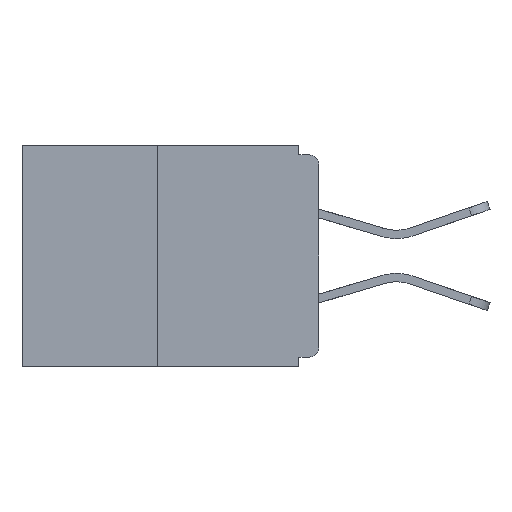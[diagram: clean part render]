
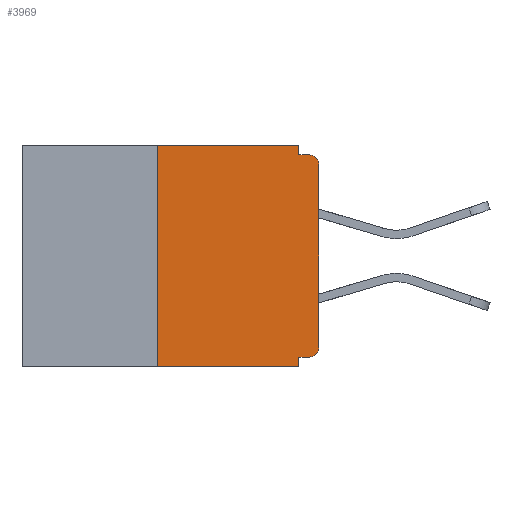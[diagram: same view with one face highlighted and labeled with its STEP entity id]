
A CAD part, left-side view. The second image highlights one B-rep face of the part: STEP entity #3969.
In plain terms, the highlighted planar face has unit normal (-1, 0, 0).
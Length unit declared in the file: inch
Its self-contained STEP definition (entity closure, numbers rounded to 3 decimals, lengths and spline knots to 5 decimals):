
#8 = VERTEX_POINT ( 'NONE', #7921 ) ;
#46 = ORIENTED_EDGE ( 'NONE', *, *, #6906, .F. ) ;
#98 = EDGE_CURVE ( 'NONE', #11477, #3747, #10595, .T. ) ;
#125 = VECTOR ( 'NONE', #12243, 39.37008 ) ;
#426 = DIRECTION ( 'NONE',  ( 0., 0., -1. ) ) ;
#535 = VERTEX_POINT ( 'NONE', #3699 ) ;
#546 = CARTESIAN_POINT ( 'NONE',  ( 0., 0.25, -0.343 ) ) ;
#581 = LINE ( 'NONE', #2381, #2431 ) ;
#599 = ORIENTED_EDGE ( 'NONE', *, *, #8883, .T. ) ;
#720 = EDGE_LOOP ( 'NONE', ( #8506, #5091, #4333, #13013, #10752, #8217, #8683, #599, #46, #11203 ) ) ;
#773 = CARTESIAN_POINT ( 'NONE',  ( 0., 0.25, 0. ) ) ;
#1029 = VECTOR ( 'NONE', #7356, 39.37008 ) ;
#1056 = CARTESIAN_POINT ( 'NONE',  ( 0., 0.46, 0. ) ) ;
#1075 = VECTOR ( 'NONE', #1654, 39.37008 ) ;
#1450 = LINE ( 'NONE', #6762, #2303 ) ;
#1654 = DIRECTION ( 'NONE',  ( 0., 0., -1. ) ) ;
#1797 = AXIS2_PLACEMENT_3D ( 'NONE', #3157, #8465, #10649 ) ;
#2116 = DIRECTION ( 'NONE',  ( -1., 0., 0. ) ) ;
#2211 = CARTESIAN_POINT ( 'NONE',  ( 0., 0.015, -0.03 ) ) ;
#2303 = VECTOR ( 'NONE', #5671, 39.37008 ) ;
#2381 = CARTESIAN_POINT ( 'NONE',  ( 0., 0.46, 0. ) ) ;
#2431 = VECTOR ( 'NONE', #8765, 39.37008 ) ;
#2503 = AXIS2_PLACEMENT_3D ( 'NONE', #1056, #4284, #10712 ) ;
#2799 = EDGE_CURVE ( 'NONE', #5408, #12318, #581, .T. ) ;
#3157 = CARTESIAN_POINT ( 'NONE',  ( 0., 0.015, -0.313 ) ) ;
#3571 = VECTOR ( 'NONE', #8159, 39.37008 ) ;
#3699 = CARTESIAN_POINT ( 'NONE',  ( 0., 0.031, -0.343 ) ) ;
#3747 = VERTEX_POINT ( 'NONE', #12670 ) ;
#3969 = ADVANCED_FACE ( 'NONE', ( #12938 ), #10816, .F. ) ;
#4093 = CARTESIAN_POINT ( 'NONE',  ( 0., 0.031, -0.328 ) ) ;
#4284 = DIRECTION ( 'NONE',  ( 1., 0., 0. ) ) ;
#4333 = ORIENTED_EDGE ( 'NONE', *, *, #10765, .T. ) ;
#4395 = DIRECTION ( 'NONE',  ( 0., 0., -1. ) ) ;
#4459 = AXIS2_PLACEMENT_3D ( 'NONE', #2211, #2116, #4395 ) ;
#4701 = CARTESIAN_POINT ( 'NONE',  ( 0., 0.015, -0.015 ) ) ;
#4711 = EDGE_CURVE ( 'NONE', #6482, #535, #12909, .T. ) ;
#4891 = CARTESIAN_POINT ( 'NONE',  ( 0., 0., 0. ) ) ;
#5045 = CIRCLE ( 'NONE', #4459, 0.015 ) ;
#5091 = ORIENTED_EDGE ( 'NONE', *, *, #6519, .F. ) ;
#5249 = DIRECTION ( 'NONE',  ( 0., 0., 1. ) ) ;
#5408 = VERTEX_POINT ( 'NONE', #773 ) ;
#5530 = LINE ( 'NONE', #6196, #8367 ) ;
#5671 = DIRECTION ( 'NONE',  ( 0., -1., 0. ) ) ;
#6196 = CARTESIAN_POINT ( 'NONE',  ( 0., 0.25, 0. ) ) ;
#6482 = VERTEX_POINT ( 'NONE', #4093 ) ;
#6519 = EDGE_CURVE ( 'NONE', #11495, #5408, #5530, .T. ) ;
#6762 = CARTESIAN_POINT ( 'NONE',  ( 0., 0.46, -0.343 ) ) ;
#6906 = EDGE_CURVE ( 'NONE', #8, #9247, #12513, .T. ) ;
#7252 = VECTOR ( 'NONE', #426, 39.37008 ) ;
#7356 = DIRECTION ( 'NONE',  ( 0., 1., 0. ) ) ;
#7921 = CARTESIAN_POINT ( 'NONE',  ( 0., 0.031, -0.015 ) ) ;
#8069 = CARTESIAN_POINT ( 'NONE',  ( 0., 0.031, 0. ) ) ;
#8094 = LINE ( 'NONE', #11783, #1029 ) ;
#8159 = DIRECTION ( 'NONE',  ( 0., 0., 1. ) ) ;
#8217 = ORIENTED_EDGE ( 'NONE', *, *, #13290, .T. ) ;
#8367 = VECTOR ( 'NONE', #5249, 39.37008 ) ;
#8465 = DIRECTION ( 'NONE',  ( -1., 0., 0. ) ) ;
#8506 = ORIENTED_EDGE ( 'NONE', *, *, #2799, .F. ) ;
#8683 = ORIENTED_EDGE ( 'NONE', *, *, #98, .T. ) ;
#8765 = DIRECTION ( 'NONE',  ( 0., -1., 0. ) ) ;
#8883 = EDGE_CURVE ( 'NONE', #3747, #9247, #5045, .T. ) ;
#8965 = CARTESIAN_POINT ( 'NONE',  ( 0., 0.031, -0.343 ) ) ;
#8981 = VERTEX_POINT ( 'NONE', #11478 ) ;
#9143 = LINE ( 'NONE', #8069, #1075 ) ;
#9247 = VERTEX_POINT ( 'NONE', #4701 ) ;
#10492 = CIRCLE ( 'NONE', #1797, 0.015 ) ;
#10595 = LINE ( 'NONE', #4891, #3571 ) ;
#10649 = DIRECTION ( 'NONE',  ( 0., 0., -1. ) ) ;
#10712 = DIRECTION ( 'NONE',  ( 0., 0., -1. ) ) ;
#10752 = ORIENTED_EDGE ( 'NONE', *, *, #12828, .F. ) ;
#10765 = EDGE_CURVE ( 'NONE', #11495, #535, #1450, .T. ) ;
#10816 = PLANE ( 'NONE',  #2503 ) ;
#11172 = CARTESIAN_POINT ( 'NONE',  ( 0., 0., -0.015 ) ) ;
#11203 = ORIENTED_EDGE ( 'NONE', *, *, #11877, .F. ) ;
#11477 = VERTEX_POINT ( 'NONE', #13274 ) ;
#11478 = CARTESIAN_POINT ( 'NONE',  ( 0., 0.015, -0.328 ) ) ;
#11495 = VERTEX_POINT ( 'NONE', #546 ) ;
#11783 = CARTESIAN_POINT ( 'NONE',  ( 0., 0., -0.328 ) ) ;
#11877 = EDGE_CURVE ( 'NONE', #12318, #8, #9143, .T. ) ;
#12243 = DIRECTION ( 'NONE',  ( 0., -1., 0. ) ) ;
#12318 = VERTEX_POINT ( 'NONE', #13042 ) ;
#12513 = LINE ( 'NONE', #11172, #125 ) ;
#12670 = CARTESIAN_POINT ( 'NONE',  ( 0., 0., -0.03 ) ) ;
#12828 = EDGE_CURVE ( 'NONE', #8981, #6482, #8094, .T. ) ;
#12909 = LINE ( 'NONE', #8965, #7252 ) ;
#12938 = FACE_OUTER_BOUND ( 'NONE', #720, .T. ) ;
#13013 = ORIENTED_EDGE ( 'NONE', *, *, #4711, .F. ) ;
#13042 = CARTESIAN_POINT ( 'NONE',  ( 0., 0.031, 0. ) ) ;
#13274 = CARTESIAN_POINT ( 'NONE',  ( 0., 0., -0.313 ) ) ;
#13290 = EDGE_CURVE ( 'NONE', #8981, #11477, #10492, .T. ) ;
